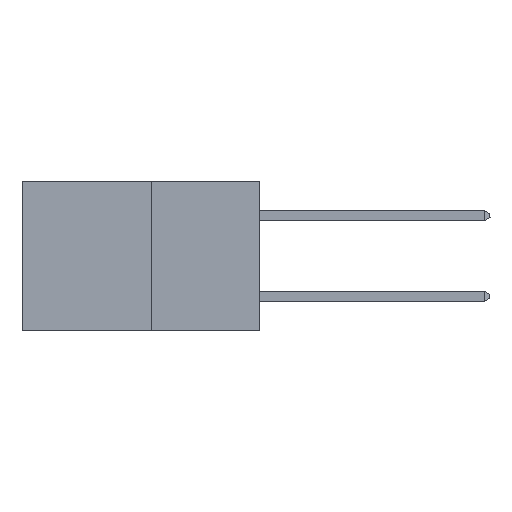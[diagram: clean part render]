
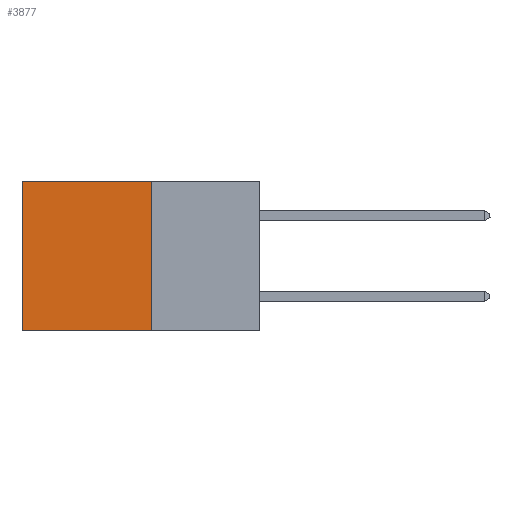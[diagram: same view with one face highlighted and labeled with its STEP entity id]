
A CAD part, left-side view. The second image highlights one B-rep face of the part: STEP entity #3877.
In plain terms, the highlighted planar face has unit normal (-1, 0, 0).
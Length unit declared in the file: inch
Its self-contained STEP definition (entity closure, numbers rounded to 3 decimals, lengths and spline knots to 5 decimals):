
#143 = EDGE_CURVE ( 'NONE', #6089, #2811, #16128, .T. ) ;
#355 = VECTOR ( 'NONE', #11292, 39.37008 ) ;
#611 = VERTEX_POINT ( 'NONE', #14980 ) ;
#1671 = DIRECTION ( 'NONE',  ( 0., 1., 0. ) ) ;
#1863 = CARTESIAN_POINT ( 'NONE',  ( 0.277, 0.27, 0. ) ) ;
#2811 = VERTEX_POINT ( 'NONE', #9783 ) ;
#3582 = LINE ( 'NONE', #11319, #355 ) ;
#3877 = ADVANCED_FACE ( 'NONE', ( #12358 ), #4971, .F. ) ;
#4010 = CARTESIAN_POINT ( 'NONE',  ( 0.277, 0.27, -0.37 ) ) ;
#4366 = DIRECTION ( 'NONE',  ( 0., 0., -1. ) ) ;
#4452 = DIRECTION ( 'NONE',  ( 1., 0., 0. ) ) ;
#4971 = PLANE ( 'NONE',  #13144 ) ;
#6080 = LINE ( 'NONE', #8586, #12221 ) ;
#6089 = VERTEX_POINT ( 'NONE', #14208 ) ;
#6851 = VECTOR ( 'NONE', #9700, 39.37008 ) ;
#8487 = DIRECTION ( 'NONE',  ( 0., 1., 0. ) ) ;
#8586 = CARTESIAN_POINT ( 'NONE',  ( 0.277, 0.27, -0.37 ) ) ;
#9700 = DIRECTION ( 'NONE',  ( 0., 0., -1. ) ) ;
#9746 = CARTESIAN_POINT ( 'NONE',  ( 0.277, 0.59, -0.37 ) ) ;
#9783 = CARTESIAN_POINT ( 'NONE',  ( 0.277, 0.59, 0. ) ) ;
#10132 = LINE ( 'NONE', #9746, #6851 ) ;
#10186 = EDGE_CURVE ( 'NONE', #6089, #13956, #3582, .T. ) ;
#11292 = DIRECTION ( 'NONE',  ( 0., 0., -1. ) ) ;
#11319 = CARTESIAN_POINT ( 'NONE',  ( 0.277, 0.27, -0.37 ) ) ;
#11578 = ORIENTED_EDGE ( 'NONE', *, *, #143, .T. ) ;
#12221 = VECTOR ( 'NONE', #8487, 39.37008 ) ;
#12358 = FACE_OUTER_BOUND ( 'NONE', #14375, .T. ) ;
#12589 = EDGE_CURVE ( 'NONE', #2811, #611, #10132, .T. ) ;
#12638 = EDGE_CURVE ( 'NONE', #13956, #611, #6080, .T. ) ;
#13029 = VECTOR ( 'NONE', #1671, 39.37008 ) ;
#13144 = AXIS2_PLACEMENT_3D ( 'NONE', #4010, #4452, #4366 ) ;
#13750 = ORIENTED_EDGE ( 'NONE', *, *, #10186, .F. ) ;
#13956 = VERTEX_POINT ( 'NONE', #15092 ) ;
#14208 = CARTESIAN_POINT ( 'NONE',  ( 0.277, 0.27, 0. ) ) ;
#14225 = ORIENTED_EDGE ( 'NONE', *, *, #12638, .F. ) ;
#14375 = EDGE_LOOP ( 'NONE', ( #15706, #14225, #13750, #11578 ) ) ;
#14980 = CARTESIAN_POINT ( 'NONE',  ( 0.277, 0.59, -0.37 ) ) ;
#15092 = CARTESIAN_POINT ( 'NONE',  ( 0.277, 0.27, -0.37 ) ) ;
#15706 = ORIENTED_EDGE ( 'NONE', *, *, #12589, .T. ) ;
#16128 = LINE ( 'NONE', #1863, #13029 ) ;
